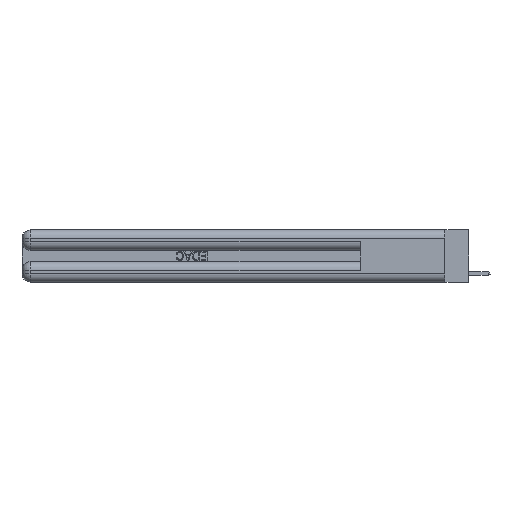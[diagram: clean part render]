
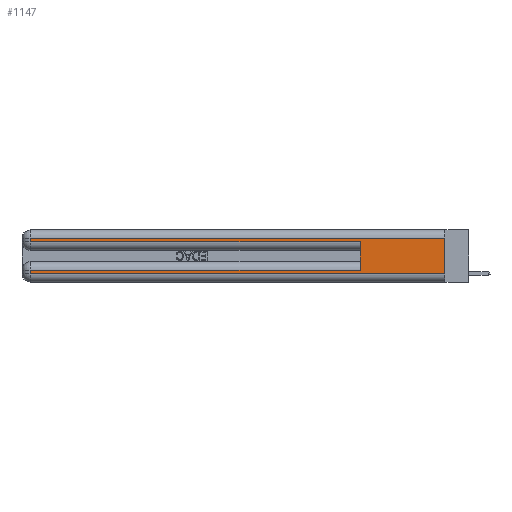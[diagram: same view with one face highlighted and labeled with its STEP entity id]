
A CAD part, left-side view. The second image highlights one B-rep face of the part: STEP entity #1147.
In plain terms, the highlighted planar face has unit normal (-1, 0, 0).
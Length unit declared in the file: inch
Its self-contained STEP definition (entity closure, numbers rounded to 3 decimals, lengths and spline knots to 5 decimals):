
#271 = EDGE_CURVE ( 'NONE', #12950, #24580, #20364, .T. ) ;
#1083 = DIRECTION ( 'NONE',  ( 0., -1., 0. ) ) ;
#1147 = ADVANCED_FACE ( 'NONE', ( #12594 ), #19966, .F. ) ;
#1444 = AXIS2_PLACEMENT_3D ( 'NONE', #27369, #5311, #24948 ) ;
#2165 = VERTEX_POINT ( 'NONE', #26472 ) ;
#4555 = CARTESIAN_POINT ( 'NONE',  ( 0., 0.6, 0.145 ) ) ;
#5134 = EDGE_CURVE ( 'NONE', #13766, #12950, #16201, .T. ) ;
#5311 = DIRECTION ( 'NONE',  ( 1., 0., 0. ) ) ;
#5404 = ORIENTED_EDGE ( 'NONE', *, *, #6142, .F. ) ;
#6142 = EDGE_CURVE ( 'NONE', #17222, #24580, #12145, .T. ) ;
#6355 = VECTOR ( 'NONE', #16357, 39.37008 ) ;
#6436 = EDGE_LOOP ( 'NONE', ( #5404, #18753, #8443, #13484, #27434, #21431, #31732, #25645 ) ) ;
#6489 = LINE ( 'NONE', #4555, #20502 ) ;
#7305 = CARTESIAN_POINT ( 'NONE',  ( 0., 2.94, 0.085 ) ) ;
#8339 = EDGE_CURVE ( 'NONE', #16706, #13849, #6489, .T. ) ;
#8443 = ORIENTED_EDGE ( 'NONE', *, *, #13871, .T. ) ;
#8638 = LINE ( 'NONE', #13495, #15175 ) ;
#9578 = DIRECTION ( 'NONE',  ( 0., 0., 1. ) ) ;
#10370 = LINE ( 'NONE', #15045, #16328 ) ;
#10885 = CARTESIAN_POINT ( 'NONE',  ( 0., 0., 0.06 ) ) ;
#11416 = DIRECTION ( 'NONE',  ( 0., 1., 0. ) ) ;
#12145 = LINE ( 'NONE', #15037, #19332 ) ;
#12594 = FACE_OUTER_BOUND ( 'NONE', #6436, .T. ) ;
#12751 = CARTESIAN_POINT ( 'NONE',  ( 0., 2.94, 0.06 ) ) ;
#12950 = VERTEX_POINT ( 'NONE', #12751 ) ;
#13484 = ORIENTED_EDGE ( 'NONE', *, *, #27767, .T. ) ;
#13495 = CARTESIAN_POINT ( 'NONE',  ( 0., 0., 0.285 ) ) ;
#13766 = VERTEX_POINT ( 'NONE', #7305 ) ;
#13849 = VERTEX_POINT ( 'NONE', #22587 ) ;
#13871 = EDGE_CURVE ( 'NONE', #2165, #24931, #10370, .T. ) ;
#14670 = VECTOR ( 'NONE', #11416, 39.37008 ) ;
#15037 = CARTESIAN_POINT ( 'NONE',  ( 0., 0., 0.37 ) ) ;
#15045 = CARTESIAN_POINT ( 'NONE',  ( 0., 2.94, 0.37 ) ) ;
#15175 = VECTOR ( 'NONE', #1083, 39.37008 ) ;
#15407 = CARTESIAN_POINT ( 'NONE',  ( 0., 0.6, 0.085 ) ) ;
#16201 = LINE ( 'NONE', #18613, #6355 ) ;
#16328 = VECTOR ( 'NONE', #22271, 39.37008 ) ;
#16357 = DIRECTION ( 'NONE',  ( 0., 0., -1. ) ) ;
#16706 = VERTEX_POINT ( 'NONE', #15407 ) ;
#17222 = VERTEX_POINT ( 'NONE', #23838 ) ;
#18353 = CARTESIAN_POINT ( 'NONE',  ( 0., 0., 0.31 ) ) ;
#18613 = CARTESIAN_POINT ( 'NONE',  ( 0., 2.94, 0.37 ) ) ;
#18721 = EDGE_CURVE ( 'NONE', #17222, #2165, #28476, .T. ) ;
#18753 = ORIENTED_EDGE ( 'NONE', *, *, #18721, .T. ) ;
#19332 = VECTOR ( 'NONE', #19367, 39.37008 ) ;
#19367 = DIRECTION ( 'NONE',  ( 0., 0., -1. ) ) ;
#19941 = VECTOR ( 'NONE', #25192, 39.37008 ) ;
#19966 = PLANE ( 'NONE',  #1444 ) ;
#20364 = LINE ( 'NONE', #10885, #19941 ) ;
#20502 = VECTOR ( 'NONE', #9578, 39.37008 ) ;
#21431 = ORIENTED_EDGE ( 'NONE', *, *, #26238, .T. ) ;
#22271 = DIRECTION ( 'NONE',  ( 0., 0., -1. ) ) ;
#22587 = CARTESIAN_POINT ( 'NONE',  ( 0., 0.6, 0.285 ) ) ;
#23838 = CARTESIAN_POINT ( 'NONE',  ( 0., 0., 0.31 ) ) ;
#24580 = VERTEX_POINT ( 'NONE', #28635 ) ;
#24931 = VERTEX_POINT ( 'NONE', #28436 ) ;
#24948 = DIRECTION ( 'NONE',  ( 0., 0., -1. ) ) ;
#25192 = DIRECTION ( 'NONE',  ( 0., -1., 0. ) ) ;
#25645 = ORIENTED_EDGE ( 'NONE', *, *, #271, .T. ) ;
#26238 = EDGE_CURVE ( 'NONE', #16706, #13766, #30891, .T. ) ;
#26472 = CARTESIAN_POINT ( 'NONE',  ( 0., 2.94, 0.31 ) ) ;
#27369 = CARTESIAN_POINT ( 'NONE',  ( 0., 0., 0.37 ) ) ;
#27434 = ORIENTED_EDGE ( 'NONE', *, *, #8339, .F. ) ;
#27767 = EDGE_CURVE ( 'NONE', #24931, #13849, #8638, .T. ) ;
#28436 = CARTESIAN_POINT ( 'NONE',  ( 0., 2.94, 0.285 ) ) ;
#28445 = CARTESIAN_POINT ( 'NONE',  ( 0., 0., 0.085 ) ) ;
#28476 = LINE ( 'NONE', #18353, #29855 ) ;
#28635 = CARTESIAN_POINT ( 'NONE',  ( 0., 0., 0.06 ) ) ;
#29855 = VECTOR ( 'NONE', #30918, 39.37008 ) ;
#30891 = LINE ( 'NONE', #28445, #14670 ) ;
#30918 = DIRECTION ( 'NONE',  ( 0., 1., 0. ) ) ;
#31732 = ORIENTED_EDGE ( 'NONE', *, *, #5134, .T. ) ;
